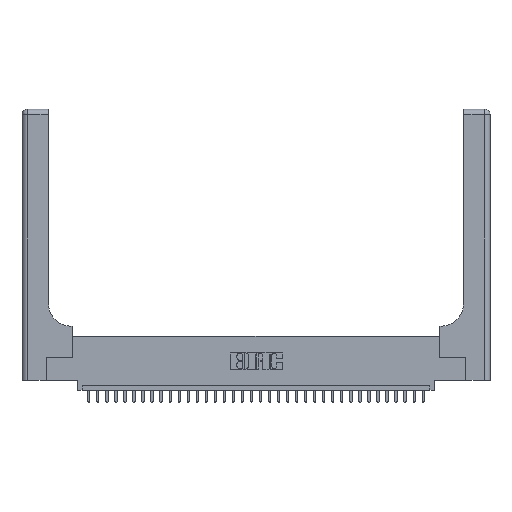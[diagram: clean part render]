
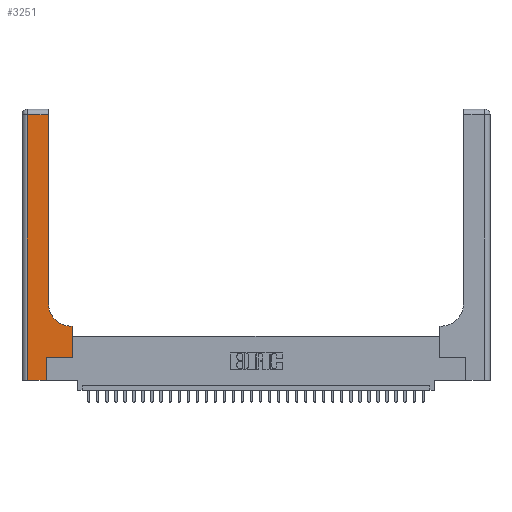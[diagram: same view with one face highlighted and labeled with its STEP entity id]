
A CAD part, top view. The second image highlights one B-rep face of the part: STEP entity #3251.
In plain terms, the highlighted planar face has unit normal (0, 0, 1).
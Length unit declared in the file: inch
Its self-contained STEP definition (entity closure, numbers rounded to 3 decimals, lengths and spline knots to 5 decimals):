
#1300 = VERTEX_POINT ( 'NONE', #21848 ) ;
#1498 = VECTOR ( 'NONE', #17285, 39.37008 ) ;
#1816 = ORIENTED_EDGE ( 'NONE', *, *, #25118, .T. ) ;
#2330 = DIRECTION ( 'NONE',  ( 0., 0., -1. ) ) ;
#2624 = EDGE_CURVE ( 'NONE', #33368, #1300, #24360, .T. ) ;
#3153 = FACE_OUTER_BOUND ( 'NONE', #18334, .T. ) ;
#3251 = ADVANCED_FACE ( 'NONE', ( #3153 ), #4511, .F. ) ;
#4511 = PLANE ( 'NONE',  #8094 ) ;
#4629 = DIRECTION ( 'NONE',  ( 0., 0., -1. ) ) ;
#4631 = ORIENTED_EDGE ( 'NONE', *, *, #22609, .T. ) ;
#4886 = CARTESIAN_POINT ( 'NONE',  ( 0.269, 0., 0.37 ) ) ;
#5538 = CARTESIAN_POINT ( 'NONE',  ( 0., 0., 0.37 ) ) ;
#5640 = DIRECTION ( 'NONE',  ( 1., 0., 0. ) ) ;
#5700 = VECTOR ( 'NONE', #30565, 39.37008 ) ;
#5941 = LINE ( 'NONE', #5538, #33366 ) ;
#7096 = VERTEX_POINT ( 'NONE', #21682 ) ;
#8032 = VECTOR ( 'NONE', #13083, 39.37008 ) ;
#8094 = AXIS2_PLACEMENT_3D ( 'NONE', #30992, #4629, #14954 ) ;
#8475 = CARTESIAN_POINT ( 'NONE',  ( 0.269, 0., 0.37 ) ) ;
#8998 = CARTESIAN_POINT ( 'NONE',  ( 0.2915, 3., 0.37 ) ) ;
#9001 = CARTESIAN_POINT ( 'NONE',  ( 0.2915, 0.85, 0.37 ) ) ;
#9446 = LINE ( 'NONE', #11945, #1498 ) ;
#10687 = VECTOR ( 'NONE', #24488, 39.37008 ) ;
#10738 = EDGE_CURVE ( 'NONE', #30357, #18564, #12910, .T. ) ;
#11281 = CARTESIAN_POINT ( 'NONE',  ( 0.2915, 0.6, 0.37 ) ) ;
#11945 = CARTESIAN_POINT ( 'NONE',  ( 0.5585, 0.25, 0.37 ) ) ;
#11971 = VERTEX_POINT ( 'NONE', #24262 ) ;
#11981 = CARTESIAN_POINT ( 'NONE',  ( 0.5585, 0.6, 0.37 ) ) ;
#12692 = CARTESIAN_POINT ( 'NONE',  ( 0.269, 0.25, 0.37 ) ) ;
#12910 = LINE ( 'NONE', #8998, #29098 ) ;
#12928 = DIRECTION ( 'NONE',  ( 1., 0., 0. ) ) ;
#13083 = DIRECTION ( 'NONE',  ( -1., 0., 0. ) ) ;
#14045 = VERTEX_POINT ( 'NONE', #22430 ) ;
#14733 = EDGE_CURVE ( 'NONE', #18564, #11971, #24188, .T. ) ;
#14954 = DIRECTION ( 'NONE',  ( -1., 0., 0. ) ) ;
#15054 = EDGE_CURVE ( 'NONE', #1300, #30357, #22110, .T. ) ;
#15118 = ORIENTED_EDGE ( 'NONE', *, *, #10738, .T. ) ;
#15753 = DIRECTION ( 'NONE',  ( 1., 0., 0. ) ) ;
#15861 = ORIENTED_EDGE ( 'NONE', *, *, #14733, .T. ) ;
#16107 = VECTOR ( 'NONE', #15753, 39.37008 ) ;
#17063 = CARTESIAN_POINT ( 'NONE',  ( 0.06, 3., 0.37 ) ) ;
#17285 = DIRECTION ( 'NONE',  ( 0., 1., 0. ) ) ;
#17739 = LINE ( 'NONE', #17063, #10687 ) ;
#17881 = VERTEX_POINT ( 'NONE', #12692 ) ;
#18322 = DIRECTION ( 'NONE',  ( 0., 1., 0. ) ) ;
#18334 = EDGE_LOOP ( 'NONE', ( #15118, #15861, #26528, #1816, #32348, #23680, #4631, #21791, #33831 ) ) ;
#18403 = CARTESIAN_POINT ( 'NONE',  ( 0.269, 0.25, 0.37 ) ) ;
#18564 = VERTEX_POINT ( 'NONE', #23432 ) ;
#18793 = EDGE_CURVE ( 'NONE', #11971, #7096, #17739, .T. ) ;
#21682 = CARTESIAN_POINT ( 'NONE',  ( 0.06, 0., 0.37 ) ) ;
#21791 = ORIENTED_EDGE ( 'NONE', *, *, #2624, .T. ) ;
#21848 = CARTESIAN_POINT ( 'NONE',  ( 0.5415, 0.6, 0.37 ) ) ;
#22110 = CIRCLE ( 'NONE', #31347, 0.25 ) ;
#22430 = CARTESIAN_POINT ( 'NONE',  ( 0.5585, 0.25, 0.37 ) ) ;
#22600 = VECTOR ( 'NONE', #18322, 39.37008 ) ;
#22609 = EDGE_CURVE ( 'NONE', #14045, #33368, #9446, .T. ) ;
#22748 = EDGE_CURVE ( 'NONE', #26276, #17881, #32618, .T. ) ;
#23432 = CARTESIAN_POINT ( 'NONE',  ( 0.2915, 2.94, 0.37 ) ) ;
#23680 = ORIENTED_EDGE ( 'NONE', *, *, #34011, .T. ) ;
#24188 = LINE ( 'NONE', #26774, #8032 ) ;
#24262 = CARTESIAN_POINT ( 'NONE',  ( 0.06, 2.94, 0.37 ) ) ;
#24360 = LINE ( 'NONE', #11281, #5700 ) ;
#24488 = DIRECTION ( 'NONE',  ( 0., -1., 0. ) ) ;
#25118 = EDGE_CURVE ( 'NONE', #7096, #26276, #5941, .T. ) ;
#25229 = LINE ( 'NONE', #18403, #16107 ) ;
#26276 = VERTEX_POINT ( 'NONE', #8475 ) ;
#26528 = ORIENTED_EDGE ( 'NONE', *, *, #18793, .T. ) ;
#26774 = CARTESIAN_POINT ( 'NONE',  ( 0., 2.94, 0.37 ) ) ;
#27422 = DIRECTION ( 'NONE',  ( 0., 1., 0. ) ) ;
#28837 = CARTESIAN_POINT ( 'NONE',  ( 0.5415, 0.85, 0.37 ) ) ;
#29098 = VECTOR ( 'NONE', #27422, 39.37008 ) ;
#30357 = VERTEX_POINT ( 'NONE', #9001 ) ;
#30565 = DIRECTION ( 'NONE',  ( -1., 0., 0. ) ) ;
#30992 = CARTESIAN_POINT ( 'NONE',  ( 0., 3., 0.37 ) ) ;
#31347 = AXIS2_PLACEMENT_3D ( 'NONE', #28837, #2330, #12928 ) ;
#32348 = ORIENTED_EDGE ( 'NONE', *, *, #22748, .T. ) ;
#32618 = LINE ( 'NONE', #4886, #22600 ) ;
#33366 = VECTOR ( 'NONE', #5640, 39.37008 ) ;
#33368 = VERTEX_POINT ( 'NONE', #11981 ) ;
#33831 = ORIENTED_EDGE ( 'NONE', *, *, #15054, .T. ) ;
#34011 = EDGE_CURVE ( 'NONE', #17881, #14045, #25229, .T. ) ;
